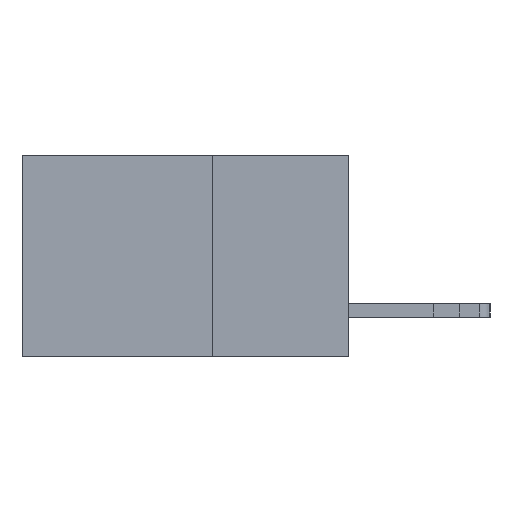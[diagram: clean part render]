
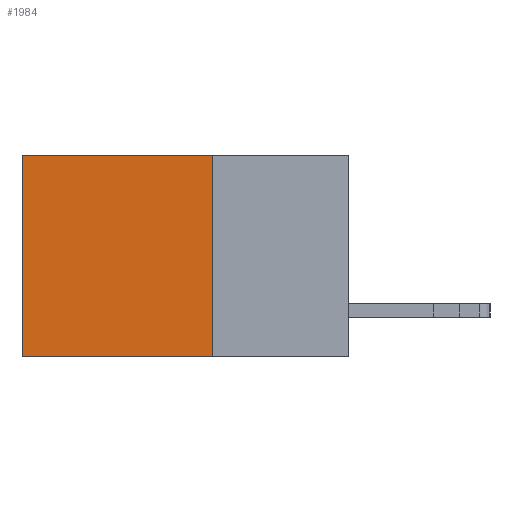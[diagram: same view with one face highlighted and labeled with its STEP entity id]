
A CAD part, left-side view. The second image highlights one B-rep face of the part: STEP entity #1984.
In plain terms, the highlighted planar face has unit normal (-1, 0, 0).
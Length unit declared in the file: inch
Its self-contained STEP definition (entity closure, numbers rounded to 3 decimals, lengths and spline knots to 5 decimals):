
#646 = LINE ( 'NONE', #10813, #3834 ) ;
#649 = CARTESIAN_POINT ( 'NONE',  ( 0.298, 0.25, 0. ) ) ;
#1054 = CARTESIAN_POINT ( 'NONE',  ( 0.298, 0.6, -0.37 ) ) ;
#1333 = DIRECTION ( 'NONE',  ( 0., 1., 0. ) ) ;
#1601 = EDGE_CURVE ( 'NONE', #7196, #14049, #8787, .T. ) ;
#1615 = VERTEX_POINT ( 'NONE', #12361 ) ;
#1882 = VECTOR ( 'NONE', #7944, 39.37008 ) ;
#1953 = CARTESIAN_POINT ( 'NONE',  ( 0.298, 0.25, 0. ) ) ;
#1984 = ADVANCED_FACE ( 'NONE', ( #6356 ), #7675, .F. ) ;
#2121 = DIRECTION ( 'NONE',  ( 1., 0., 0. ) ) ;
#2587 = VECTOR ( 'NONE', #11404, 39.37008 ) ;
#3834 = VECTOR ( 'NONE', #1333, 39.37008 ) ;
#4051 = EDGE_CURVE ( 'NONE', #8439, #7196, #12712, .T. ) ;
#4368 = CARTESIAN_POINT ( 'NONE',  ( 0.298, 0.6, 0. ) ) ;
#4764 = ORIENTED_EDGE ( 'NONE', *, *, #1601, .F. ) ;
#5071 = LINE ( 'NONE', #4368, #1882 ) ;
#5667 = ORIENTED_EDGE ( 'NONE', *, *, #9387, .T. ) ;
#6271 = CARTESIAN_POINT ( 'NONE',  ( 0.298, 0.25, 0. ) ) ;
#6356 = FACE_OUTER_BOUND ( 'NONE', #10520, .T. ) ;
#7196 = VERTEX_POINT ( 'NONE', #10995 ) ;
#7675 = PLANE ( 'NONE',  #8427 ) ;
#7944 = DIRECTION ( 'NONE',  ( 0., 0., -1. ) ) ;
#8427 = AXIS2_PLACEMENT_3D ( 'NONE', #6271, #2121, #10928 ) ;
#8439 = VERTEX_POINT ( 'NONE', #649 ) ;
#8787 = LINE ( 'NONE', #11358, #12221 ) ;
#9190 = DIRECTION ( 'NONE',  ( 0., 1., 0. ) ) ;
#9387 = EDGE_CURVE ( 'NONE', #1615, #14049, #5071, .T. ) ;
#10520 = EDGE_LOOP ( 'NONE', ( #5667, #4764, #14050, #11025 ) ) ;
#10813 = CARTESIAN_POINT ( 'NONE',  ( 0.298, 0.25, 0. ) ) ;
#10928 = DIRECTION ( 'NONE',  ( 0., 0., -1. ) ) ;
#10947 = EDGE_CURVE ( 'NONE', #8439, #1615, #646, .T. ) ;
#10995 = CARTESIAN_POINT ( 'NONE',  ( 0.298, 0.25, -0.37 ) ) ;
#11025 = ORIENTED_EDGE ( 'NONE', *, *, #10947, .T. ) ;
#11358 = CARTESIAN_POINT ( 'NONE',  ( 0.298, 0.25, -0.37 ) ) ;
#11404 = DIRECTION ( 'NONE',  ( 0., 0., -1. ) ) ;
#12221 = VECTOR ( 'NONE', #9190, 39.37008 ) ;
#12361 = CARTESIAN_POINT ( 'NONE',  ( 0.298, 0.6, 0. ) ) ;
#12712 = LINE ( 'NONE', #1953, #2587 ) ;
#14049 = VERTEX_POINT ( 'NONE', #1054 ) ;
#14050 = ORIENTED_EDGE ( 'NONE', *, *, #4051, .F. ) ;
